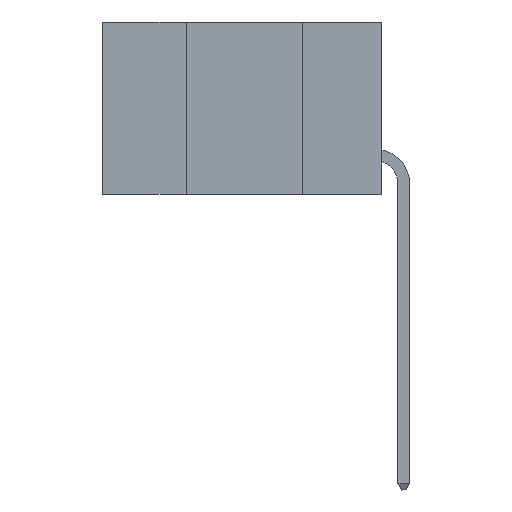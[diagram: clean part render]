
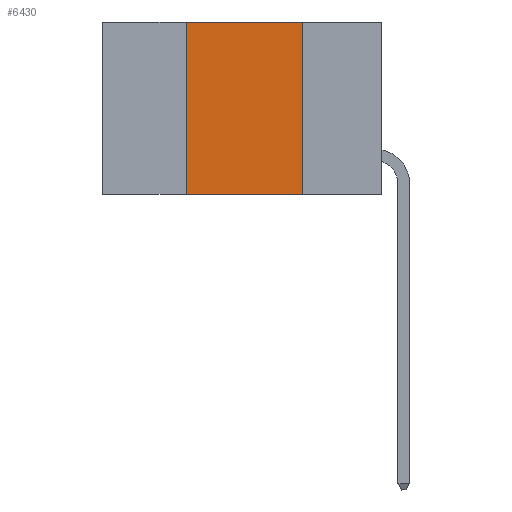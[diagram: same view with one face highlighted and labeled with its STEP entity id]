
A CAD part, left-side view. The second image highlights one B-rep face of the part: STEP entity #6430.
In plain terms, the highlighted planar face has unit normal (-1, 0, 0).
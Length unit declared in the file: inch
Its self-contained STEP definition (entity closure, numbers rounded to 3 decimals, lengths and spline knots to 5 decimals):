
#323 = EDGE_CURVE ( 'NONE', #11464, #7274, #8516, .T. ) ;
#640 = ORIENTED_EDGE ( 'NONE', *, *, #9581, .F. ) ;
#1873 = CARTESIAN_POINT ( 'NONE',  ( 0., 0.42, -0.37 ) ) ;
#2490 = VECTOR ( 'NONE', #13047, 39.37008 ) ;
#2503 = LINE ( 'NONE', #12590, #5520 ) ;
#2769 = CARTESIAN_POINT ( 'NONE',  ( 0., 0.17, 0. ) ) ;
#3313 = CARTESIAN_POINT ( 'NONE',  ( 0., 0.6, -0.37 ) ) ;
#3390 = DIRECTION ( 'NONE',  ( 0., 0., 1. ) ) ;
#3923 = VERTEX_POINT ( 'NONE', #5804 ) ;
#4428 = ORIENTED_EDGE ( 'NONE', *, *, #5054, .F. ) ;
#4514 = CARTESIAN_POINT ( 'NONE',  ( 0., 0.17, -0.37 ) ) ;
#4573 = LINE ( 'NONE', #4846, #10701 ) ;
#4684 = LINE ( 'NONE', #4828, #2490 ) ;
#4828 = CARTESIAN_POINT ( 'NONE',  ( 0., 0.6, 0. ) ) ;
#4846 = CARTESIAN_POINT ( 'NONE',  ( 0., 0.17, 0. ) ) ;
#5054 = EDGE_CURVE ( 'NONE', #3923, #11336, #4684, .T. ) ;
#5520 = VECTOR ( 'NONE', #3390, 39.37008 ) ;
#5804 = CARTESIAN_POINT ( 'NONE',  ( 0., 0.42, 0. ) ) ;
#5865 = EDGE_LOOP ( 'NONE', ( #640, #4428, #11450, #12303 ) ) ;
#6100 = FACE_OUTER_BOUND ( 'NONE', #5865, .T. ) ;
#6430 = ADVANCED_FACE ( 'NONE', ( #6100 ), #10115, .F. ) ;
#7274 = VERTEX_POINT ( 'NONE', #4514 ) ;
#7899 = DIRECTION ( 'NONE',  ( 0., 0., -1. ) ) ;
#8329 = DIRECTION ( 'NONE',  ( 0., -1., 0. ) ) ;
#8516 = LINE ( 'NONE', #3313, #11543 ) ;
#9581 = EDGE_CURVE ( 'NONE', #11336, #7274, #4573, .T. ) ;
#10019 = DIRECTION ( 'NONE',  ( 1., 0., 0. ) ) ;
#10115 = PLANE ( 'NONE',  #12643 ) ;
#10512 = EDGE_CURVE ( 'NONE', #11464, #3923, #2503, .T. ) ;
#10701 = VECTOR ( 'NONE', #13075, 39.37008 ) ;
#11336 = VERTEX_POINT ( 'NONE', #2769 ) ;
#11450 = ORIENTED_EDGE ( 'NONE', *, *, #10512, .F. ) ;
#11464 = VERTEX_POINT ( 'NONE', #1873 ) ;
#11543 = VECTOR ( 'NONE', #8329, 39.37008 ) ;
#12303 = ORIENTED_EDGE ( 'NONE', *, *, #323, .T. ) ;
#12590 = CARTESIAN_POINT ( 'NONE',  ( 0., 0.42, 0. ) ) ;
#12643 = AXIS2_PLACEMENT_3D ( 'NONE', #13146, #10019, #7899 ) ;
#13047 = DIRECTION ( 'NONE',  ( 0., -1., 0. ) ) ;
#13075 = DIRECTION ( 'NONE',  ( 0., 0., -1. ) ) ;
#13146 = CARTESIAN_POINT ( 'NONE',  ( 0., 0.6, 0. ) ) ;
